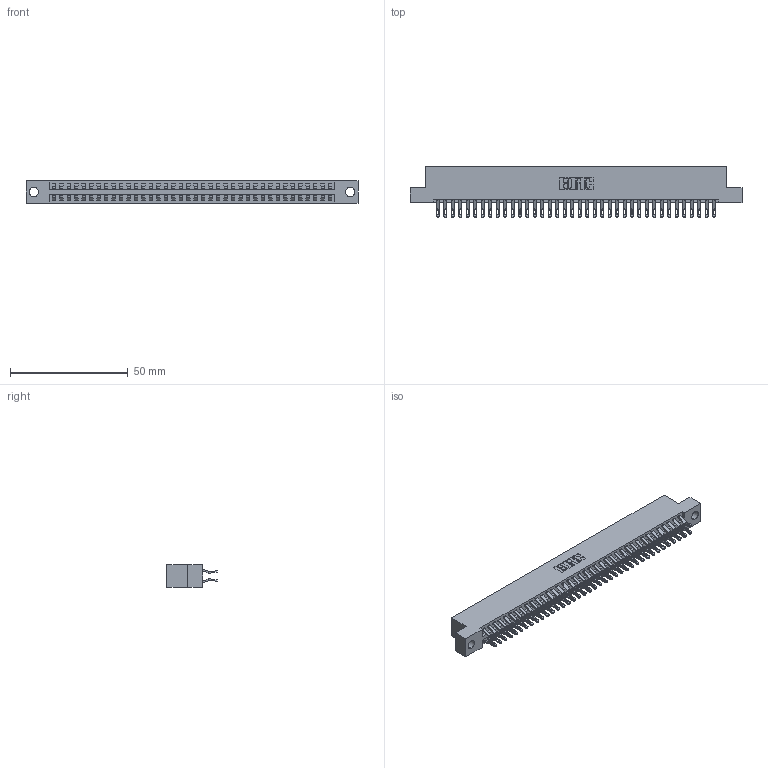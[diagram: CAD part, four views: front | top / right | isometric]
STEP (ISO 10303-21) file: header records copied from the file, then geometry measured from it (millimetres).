
FILE_DESCRIPTION (( 'STEP AP203' ), '1' );
FILE_NAME ('396-076-555-204.STEP', '2019-10-30T21:33:18', ( '' ), ( '' ), 'SwSTEP 2.0', 'SolidWorks 2016', '' );
FILE_SCHEMA (( 'CONFIG_CONTROL_DESIGN' ));
Length unit declared in the file: inch
Products named in the file (3): 345-292-001_555 Tail; 346 Part_Flush Mounting Lugs - 0.156 Dia-TH; 396-076-555-204
Assembly tree (77 placements, depth 2):
  396-076-555-204
    346 Part_Flush Mounting Lugs - 0.156 Dia-TH
    345-292-001_555 Tail  x76
Bounding box: 141.22 x 21.46 x 9.4 mm (x, y, z)
Volume: 13872.6 mm3; surface area: 19605.1 mm2
Topology: 77 solids, 77 shells, 4530 faces, 14237 edges, 9490 vertices
Faces by surface type: plane 2584, cylinder 1946
Entity records: 25667 total; most frequent: CARTESIAN_POINT 4270, ORIENTED_EDGE 4174, DIRECTION 3783, EDGE_CURVE 2087, LINE 1783, VECTOR 1783, VERTEX_POINT 1390, AXIS2_PLACEMENT_3D 1000
